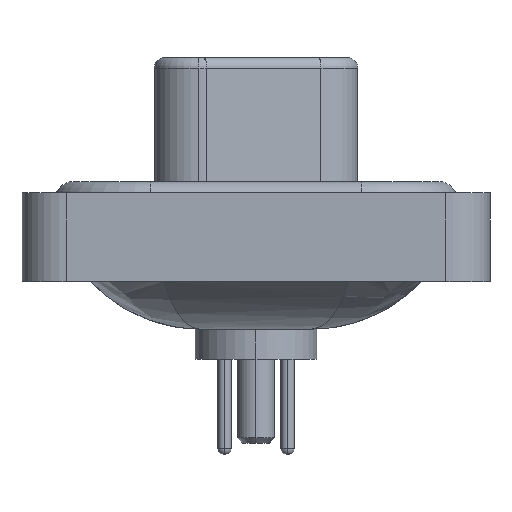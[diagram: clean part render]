
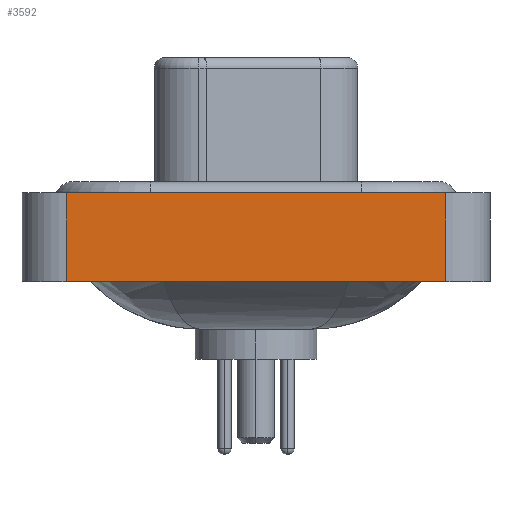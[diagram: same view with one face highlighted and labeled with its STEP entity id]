
A CAD part, left-side view. The second image highlights one B-rep face of the part: STEP entity #3592.
In plain terms, the highlighted planar face has unit normal (-1, 0, 0).
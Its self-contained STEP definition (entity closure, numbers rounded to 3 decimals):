
#509 = CARTESIAN_POINT ( 'NONE',  ( -7.35, 8.55, -3.6 ) ) ;
#537 = ORIENTED_EDGE ( 'NONE', *, *, #20878, .F. ) ;
#912 = EDGE_CURVE ( 'NONE', #12070, #17064, #14294, .T. ) ;
#1127 = ORIENTED_EDGE ( 'NONE', *, *, #912, .T. ) ;
#1627 = FACE_OUTER_BOUND ( 'NONE', #12990, .T. ) ;
#2490 = VERTEX_POINT ( 'NONE', #509 ) ;
#2835 = LINE ( 'NONE', #9567, #4668 ) ;
#3008 = VECTOR ( 'NONE', #12735, 1000. ) ;
#3592 = ADVANCED_FACE ( 'NONE', ( #1627 ), #16324, .T. ) ;
#4255 = CARTESIAN_POINT ( 'NONE',  ( -7.35, -8.55, 0.4 ) ) ;
#4417 = CARTESIAN_POINT ( 'NONE',  ( -7.35, -8.55, -3.6 ) ) ;
#4668 = VECTOR ( 'NONE', #9165, 1000. ) ;
#5438 = CARTESIAN_POINT ( 'NONE',  ( -7.35, -8.55, -3.6 ) ) ;
#6090 = AXIS2_PLACEMENT_3D ( 'NONE', #11260, #21496, #17960 ) ;
#9165 = DIRECTION ( 'NONE',  ( 0., 0., 1. ) ) ;
#9567 = CARTESIAN_POINT ( 'NONE',  ( -7.35, 8.55, -3.6 ) ) ;
#9607 = VERTEX_POINT ( 'NONE', #16050 ) ;
#10146 = EDGE_CURVE ( 'NONE', #2490, #9607, #2835, .T. ) ;
#10931 = DIRECTION ( 'NONE',  ( 0., -1., 0. ) ) ;
#11260 = CARTESIAN_POINT ( 'NONE',  ( -7.35, -8.55, -3.6 ) ) ;
#11735 = ORIENTED_EDGE ( 'NONE', *, *, #10146, .F. ) ;
#11786 = LINE ( 'NONE', #5438, #14921 ) ;
#12070 = VERTEX_POINT ( 'NONE', #16658 ) ;
#12483 = CARTESIAN_POINT ( 'NONE',  ( -7.35, -8.55, 0.4 ) ) ;
#12735 = DIRECTION ( 'NONE',  ( 0., 0., 1. ) ) ;
#12856 = ORIENTED_EDGE ( 'NONE', *, *, #19404, .T. ) ;
#12990 = EDGE_LOOP ( 'NONE', ( #1127, #537, #11735, #12856 ) ) ;
#14294 = LINE ( 'NONE', #4417, #3008 ) ;
#14921 = VECTOR ( 'NONE', #18482, 1000. ) ;
#16050 = CARTESIAN_POINT ( 'NONE',  ( -7.35, 8.55, 0.4 ) ) ;
#16324 = PLANE ( 'NONE',  #6090 ) ;
#16658 = CARTESIAN_POINT ( 'NONE',  ( -7.35, -8.55, -3.6 ) ) ;
#17064 = VERTEX_POINT ( 'NONE', #4255 ) ;
#17530 = LINE ( 'NONE', #12483, #21587 ) ;
#17960 = DIRECTION ( 'NONE',  ( 0., 0., 1. ) ) ;
#18482 = DIRECTION ( 'NONE',  ( 0., -1., 0. ) ) ;
#19404 = EDGE_CURVE ( 'NONE', #2490, #12070, #11786, .T. ) ;
#20878 = EDGE_CURVE ( 'NONE', #9607, #17064, #17530, .T. ) ;
#21496 = DIRECTION ( 'NONE',  ( -1., 0., 0. ) ) ;
#21587 = VECTOR ( 'NONE', #10931, 1000. ) ;
